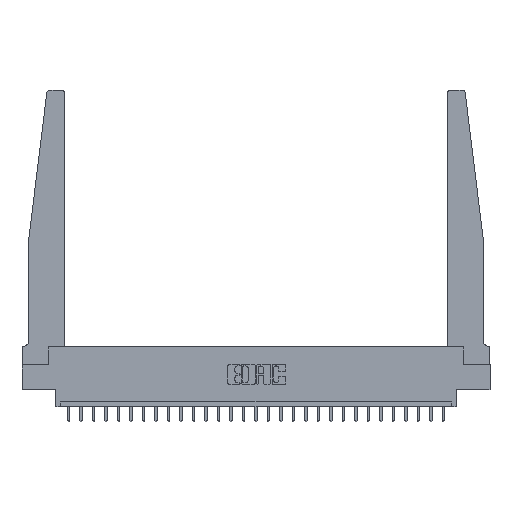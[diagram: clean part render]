
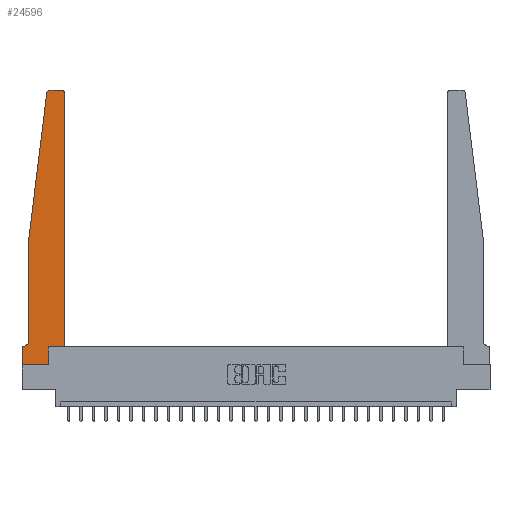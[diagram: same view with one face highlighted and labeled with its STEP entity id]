
A CAD part, top view. The second image highlights one B-rep face of the part: STEP entity #24596.
In plain terms, the highlighted planar face has unit normal (0, 0, 1).
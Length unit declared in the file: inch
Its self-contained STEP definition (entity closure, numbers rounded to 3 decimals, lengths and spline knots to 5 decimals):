
#561 = ORIENTED_EDGE ( 'NONE', *, *, #1228, .T. ) ;
#694 = CARTESIAN_POINT ( 'NONE',  ( 0.015, 0.2375, 0.37 ) ) ;
#1116 = EDGE_CURVE ( 'NONE', #11623, #14470, #15689, .T. ) ;
#1228 = EDGE_CURVE ( 'NONE', #4727, #11623, #6850, .T. ) ;
#1449 = LINE ( 'NONE', #7075, #25305 ) ;
#1802 = CARTESIAN_POINT ( 'NONE',  ( 0.015, 0.1875, 0.37 ) ) ;
#2495 = CARTESIAN_POINT ( 'NONE',  ( 0.065, 1.25, 0.37 ) ) ;
#2646 = AXIS2_PLACEMENT_3D ( 'NONE', #11293, #21073, #2992 ) ;
#2992 = DIRECTION ( 'NONE',  ( 1., 0., 0. ) ) ;
#3081 = DIRECTION ( 'NONE',  ( 0., -1., 0. ) ) ;
#3349 = VERTEX_POINT ( 'NONE', #21980 ) ;
#3698 = EDGE_CURVE ( 'NONE', #23559, #25339, #13630, .T. ) ;
#4099 = ORIENTED_EDGE ( 'NONE', *, *, #1116, .T. ) ;
#4234 = ORIENTED_EDGE ( 'NONE', *, *, #3698, .T. ) ;
#4402 = DIRECTION ( 'NONE',  ( 1., 0., 0. ) ) ;
#4727 = VERTEX_POINT ( 'NONE', #14440 ) ;
#4842 = CARTESIAN_POINT ( 'NONE',  ( 0., 0.1875, 0.37 ) ) ;
#5852 = LINE ( 'NONE', #10726, #22203 ) ;
#5984 = ORIENTED_EDGE ( 'NONE', *, *, #25162, .T. ) ;
#5999 = CARTESIAN_POINT ( 'NONE',  ( 0.2605, 0., 0.37 ) ) ;
#6325 = ORIENTED_EDGE ( 'NONE', *, *, #10835, .T. ) ;
#6641 = EDGE_LOOP ( 'NONE', ( #13986, #19315, #5984, #561, #4099, #14168, #22339, #6325, #9838, #4234, #14099, #11757 ) ) ;
#6842 = CARTESIAN_POINT ( 'NONE',  ( 0.425, 2.72, 0.37 ) ) ;
#6850 = LINE ( 'NONE', #15025, #9390 ) ;
#7075 = CARTESIAN_POINT ( 'NONE',  ( 0.065, 0.1875, 0.37 ) ) ;
#7252 = CIRCLE ( 'NONE', #2646, 0.03 ) ;
#7455 = EDGE_CURVE ( 'NONE', #19443, #7788, #7526, .T. ) ;
#7526 = LINE ( 'NONE', #21280, #24375 ) ;
#7788 = VERTEX_POINT ( 'NONE', #12925 ) ;
#8441 = DIRECTION ( 'NONE',  ( 1., 0., 0. ) ) ;
#9000 = AXIS2_PLACEMENT_3D ( 'NONE', #11043, #23572, #17374 ) ;
#9001 = VERTEX_POINT ( 'NONE', #18857 ) ;
#9266 = DIRECTION ( 'NONE',  ( 1., 0., 0. ) ) ;
#9333 = DIRECTION ( 'NONE',  ( -1., 0., 0. ) ) ;
#9390 = VECTOR ( 'NONE', #19240, 39.37008 ) ;
#9559 = LINE ( 'NONE', #12417, #13914 ) ;
#9822 = LINE ( 'NONE', #13898, #10277 ) ;
#9838 = ORIENTED_EDGE ( 'NONE', *, *, #24594, .T. ) ;
#10277 = VECTOR ( 'NONE', #25926, 39.37008 ) ;
#10312 = DIRECTION ( 'NONE',  ( 0., 1., 0. ) ) ;
#10485 = CARTESIAN_POINT ( 'NONE',  ( 0.065, 0.2375, 0.37 ) ) ;
#10538 = AXIS2_PLACEMENT_3D ( 'NONE', #19985, #22577, #8441 ) ;
#10726 = CARTESIAN_POINT ( 'NONE',  ( 0., 0., 0.37 ) ) ;
#10835 = EDGE_CURVE ( 'NONE', #7788, #21750, #5852, .T. ) ;
#11043 = CARTESIAN_POINT ( 'NONE',  ( 0.395, 2.72, 0.37 ) ) ;
#11293 = CARTESIAN_POINT ( 'NONE',  ( 0.27653, 2.72, 0.37 ) ) ;
#11329 = CARTESIAN_POINT ( 'NONE',  ( 0.425, 0.18, 0.37 ) ) ;
#11623 = VERTEX_POINT ( 'NONE', #10485 ) ;
#11757 = ORIENTED_EDGE ( 'NONE', *, *, #19168, .T. ) ;
#12417 = CARTESIAN_POINT ( 'NONE',  ( 0.2605, 0.18, 0.37 ) ) ;
#12431 = EDGE_CURVE ( 'NONE', #25339, #18557, #17533, .T. ) ;
#12925 = CARTESIAN_POINT ( 'NONE',  ( 0., 0., 0.37 ) ) ;
#13630 = LINE ( 'NONE', #25381, #16084 ) ;
#13898 = CARTESIAN_POINT ( 'NONE',  ( 0.25, 2.75, 0.37 ) ) ;
#13914 = VECTOR ( 'NONE', #10312, 39.37008 ) ;
#13986 = ORIENTED_EDGE ( 'NONE', *, *, #19707, .T. ) ;
#14099 = ORIENTED_EDGE ( 'NONE', *, *, #12431, .T. ) ;
#14168 = ORIENTED_EDGE ( 'NONE', *, *, #25376, .T. ) ;
#14440 = CARTESIAN_POINT ( 'NONE',  ( 0.065, 1.25, 0.37 ) ) ;
#14470 = VERTEX_POINT ( 'NONE', #1802 ) ;
#14516 = PLANE ( 'NONE',  #10538 ) ;
#14743 = VECTOR ( 'NONE', #24649, 39.37008 ) ;
#15025 = CARTESIAN_POINT ( 'NONE',  ( 0.065, 1.25, 0.37 ) ) ;
#15689 = CIRCLE ( 'NONE', #22423, 0.05 ) ;
#16084 = VECTOR ( 'NONE', #9266, 39.37008 ) ;
#16244 = DIRECTION ( 'NONE',  ( 0., 0., -1. ) ) ;
#16502 = FACE_OUTER_BOUND ( 'NONE', #6641, .T. ) ;
#17001 = LINE ( 'NONE', #2495, #14743 ) ;
#17374 = DIRECTION ( 'NONE',  ( 1., 0., 0. ) ) ;
#17533 = LINE ( 'NONE', #11329, #24488 ) ;
#17812 = EDGE_CURVE ( 'NONE', #3349, #25523, #7252, .T. ) ;
#18259 = CIRCLE ( 'NONE', #9000, 0.03 ) ;
#18557 = VERTEX_POINT ( 'NONE', #6842 ) ;
#18857 = CARTESIAN_POINT ( 'NONE',  ( 0.395, 2.75, 0.37 ) ) ;
#19168 = EDGE_CURVE ( 'NONE', #18557, #9001, #18259, .T. ) ;
#19220 = CARTESIAN_POINT ( 'NONE',  ( 0.425, 0.18, 0.37 ) ) ;
#19240 = DIRECTION ( 'NONE',  ( 0., -1., 0. ) ) ;
#19315 = ORIENTED_EDGE ( 'NONE', *, *, #17812, .T. ) ;
#19443 = VERTEX_POINT ( 'NONE', #4842 ) ;
#19707 = EDGE_CURVE ( 'NONE', #9001, #3349, #9822, .T. ) ;
#19985 = CARTESIAN_POINT ( 'NONE',  ( 0., 0.1875, 0.37 ) ) ;
#20195 = DIRECTION ( 'NONE',  ( -1., 0., 0. ) ) ;
#21073 = DIRECTION ( 'NONE',  ( 0., 0., 1. ) ) ;
#21280 = CARTESIAN_POINT ( 'NONE',  ( 0., 0., 0.37 ) ) ;
#21750 = VERTEX_POINT ( 'NONE', #5999 ) ;
#21980 = CARTESIAN_POINT ( 'NONE',  ( 0.27653, 2.75, 0.37 ) ) ;
#22203 = VECTOR ( 'NONE', #4402, 39.37008 ) ;
#22339 = ORIENTED_EDGE ( 'NONE', *, *, #7455, .T. ) ;
#22423 = AXIS2_PLACEMENT_3D ( 'NONE', #694, #16244, #20195 ) ;
#22577 = DIRECTION ( 'NONE',  ( 0., 0., 1. ) ) ;
#23077 = CARTESIAN_POINT ( 'NONE',  ( 0.2605, 0.18, 0.37 ) ) ;
#23559 = VERTEX_POINT ( 'NONE', #23077 ) ;
#23572 = DIRECTION ( 'NONE',  ( 0., 0., 1. ) ) ;
#24375 = VECTOR ( 'NONE', #3081, 39.37008 ) ;
#24454 = CARTESIAN_POINT ( 'NONE',  ( 0.24675, 2.72367, 0.37 ) ) ;
#24488 = VECTOR ( 'NONE', #25070, 39.37008 ) ;
#24594 = EDGE_CURVE ( 'NONE', #21750, #23559, #9559, .T. ) ;
#24596 = ADVANCED_FACE ( 'NONE', ( #16502 ), #14516, .T. ) ;
#24649 = DIRECTION ( 'NONE',  ( -0.122, -0.992, 0. ) ) ;
#25070 = DIRECTION ( 'NONE',  ( 0., 1., 0. ) ) ;
#25162 = EDGE_CURVE ( 'NONE', #25523, #4727, #17001, .T. ) ;
#25305 = VECTOR ( 'NONE', #9333, 39.37008 ) ;
#25339 = VERTEX_POINT ( 'NONE', #19220 ) ;
#25376 = EDGE_CURVE ( 'NONE', #14470, #19443, #1449, .T. ) ;
#25381 = CARTESIAN_POINT ( 'NONE',  ( 0.425, 0.18, 0.37 ) ) ;
#25523 = VERTEX_POINT ( 'NONE', #24454 ) ;
#25926 = DIRECTION ( 'NONE',  ( -1., 0., 0. ) ) ;
